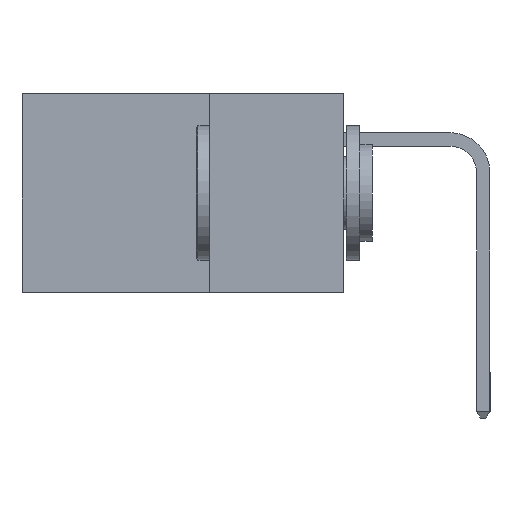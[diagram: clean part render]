
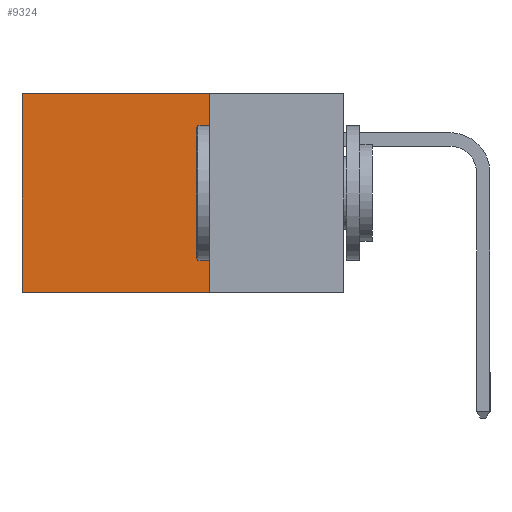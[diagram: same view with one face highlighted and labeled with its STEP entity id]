
A CAD part, left-side view. The second image highlights one B-rep face of the part: STEP entity #9324.
In plain terms, the highlighted planar face has unit normal (-1, 0, 0).
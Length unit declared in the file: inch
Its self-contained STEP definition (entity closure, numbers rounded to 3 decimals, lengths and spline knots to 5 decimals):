
#37 = LINE ( 'NONE', #11451, #30701 ) ;
#824 = DIRECTION ( 'NONE',  ( 0., 0., -1. ) ) ;
#1353 = VERTEX_POINT ( 'NONE', #13209 ) ;
#1644 = ORIENTED_EDGE ( 'NONE', *, *, #12351, .F. ) ;
#2280 = FACE_OUTER_BOUND ( 'NONE', #7064, .T. ) ;
#3040 = CARTESIAN_POINT ( 'NONE',  ( 0.298, 0.25, 0. ) ) ;
#7064 = EDGE_LOOP ( 'NONE', ( #31410, #31646, #1644, #21370 ) ) ;
#7234 = VECTOR ( 'NONE', #15287, 39.37008 ) ;
#8139 = EDGE_CURVE ( 'NONE', #15315, #1353, #37, .T. ) ;
#8308 = AXIS2_PLACEMENT_3D ( 'NONE', #18673, #8407, #824 ) ;
#8407 = DIRECTION ( 'NONE',  ( 1., 0., 0. ) ) ;
#8593 = CARTESIAN_POINT ( 'NONE',  ( 0.298, 0.25, 0. ) ) ;
#8612 = VERTEX_POINT ( 'NONE', #28977 ) ;
#9324 = ADVANCED_FACE ( 'NONE', ( #2280 ), #18455, .F. ) ;
#11120 = DIRECTION ( 'NONE',  ( 0., 1., 0. ) ) ;
#11451 = CARTESIAN_POINT ( 'NONE',  ( 0.298, 0.25, -0.37 ) ) ;
#12351 = EDGE_CURVE ( 'NONE', #25712, #15315, #13968, .T. ) ;
#13209 = CARTESIAN_POINT ( 'NONE',  ( 0.298, 0.6, -0.37 ) ) ;
#13968 = LINE ( 'NONE', #3040, #7234 ) ;
#14400 = EDGE_CURVE ( 'NONE', #8612, #1353, #23488, .T. ) ;
#15287 = DIRECTION ( 'NONE',  ( 0., 0., -1. ) ) ;
#15315 = VERTEX_POINT ( 'NONE', #32561 ) ;
#17452 = LINE ( 'NONE', #8593, #31576 ) ;
#17825 = CARTESIAN_POINT ( 'NONE',  ( 0.298, 0.25, 0. ) ) ;
#18455 = PLANE ( 'NONE',  #8308 ) ;
#18673 = CARTESIAN_POINT ( 'NONE',  ( 0.298, 0.25, 0. ) ) ;
#21370 = ORIENTED_EDGE ( 'NONE', *, *, #22677, .T. ) ;
#22677 = EDGE_CURVE ( 'NONE', #25712, #8612, #17452, .T. ) ;
#23123 = DIRECTION ( 'NONE',  ( 0., 0., -1. ) ) ;
#23488 = LINE ( 'NONE', #28029, #25800 ) ;
#25712 = VERTEX_POINT ( 'NONE', #17825 ) ;
#25800 = VECTOR ( 'NONE', #23123, 39.37008 ) ;
#28029 = CARTESIAN_POINT ( 'NONE',  ( 0.298, 0.6, 0. ) ) ;
#28977 = CARTESIAN_POINT ( 'NONE',  ( 0.298, 0.6, 0. ) ) ;
#30701 = VECTOR ( 'NONE', #31560, 39.37008 ) ;
#31410 = ORIENTED_EDGE ( 'NONE', *, *, #14400, .T. ) ;
#31560 = DIRECTION ( 'NONE',  ( 0., 1., 0. ) ) ;
#31576 = VECTOR ( 'NONE', #11120, 39.37008 ) ;
#31646 = ORIENTED_EDGE ( 'NONE', *, *, #8139, .F. ) ;
#32561 = CARTESIAN_POINT ( 'NONE',  ( 0.298, 0.25, -0.37 ) ) ;
